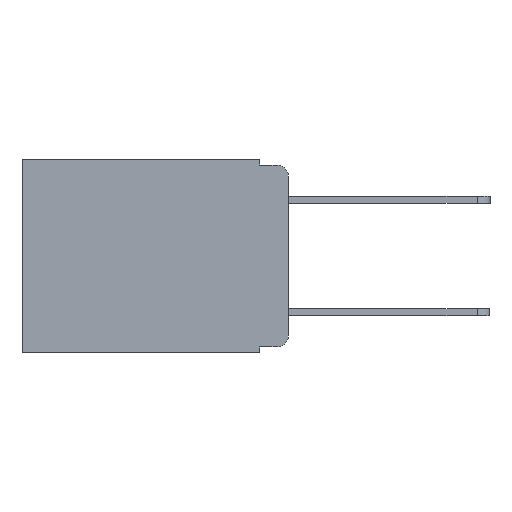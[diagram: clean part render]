
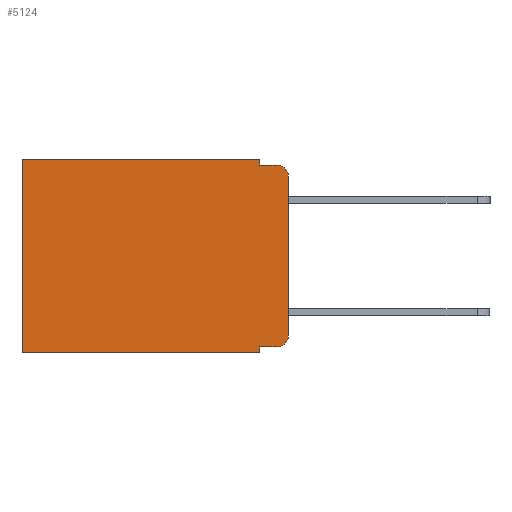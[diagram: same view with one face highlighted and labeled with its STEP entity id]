
A CAD part, left-side view. The second image highlights one B-rep face of the part: STEP entity #5124.
In plain terms, the highlighted planar face has unit normal (-1, 0, 0).
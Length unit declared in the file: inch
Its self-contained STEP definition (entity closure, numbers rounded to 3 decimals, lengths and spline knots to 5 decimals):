
#70 = LINE ( 'NONE', #1626, #19078 ) ;
#464 = ORIENTED_EDGE ( 'NONE', *, *, #7212, .F. ) ;
#590 = CARTESIAN_POINT ( 'NONE',  ( 0.298, 0., 0. ) ) ;
#934 = VERTEX_POINT ( 'NONE', #15939 ) ;
#961 = CIRCLE ( 'NONE', #19125, 0.02 ) ;
#998 = VECTOR ( 'NONE', #14916, 39.37008 ) ;
#1626 = CARTESIAN_POINT ( 'NONE',  ( 0.298, 0.051, -0.01 ) ) ;
#1987 = ORIENTED_EDGE ( 'NONE', *, *, #23330, .T. ) ;
#2326 = VECTOR ( 'NONE', #5516, 39.37008 ) ;
#2401 = CARTESIAN_POINT ( 'NONE',  ( 0.298, 0.02, -0.01 ) ) ;
#2480 = CARTESIAN_POINT ( 'NONE',  ( 0.298, 0.051, -0.343 ) ) ;
#2609 = ORIENTED_EDGE ( 'NONE', *, *, #18792, .T. ) ;
#2703 = EDGE_CURVE ( 'NONE', #2738, #21969, #961, .T. ) ;
#2738 = VERTEX_POINT ( 'NONE', #14246 ) ;
#2859 = CIRCLE ( 'NONE', #20068, 0.02 ) ;
#3215 = ORIENTED_EDGE ( 'NONE', *, *, #3689, .F. ) ;
#3340 = VECTOR ( 'NONE', #21827, 39.37008 ) ;
#3397 = EDGE_CURVE ( 'NONE', #18143, #21969, #20705, .T. ) ;
#3503 = VECTOR ( 'NONE', #4278, 39.37008 ) ;
#3689 = EDGE_CURVE ( 'NONE', #23523, #934, #20412, .T. ) ;
#3880 = ORIENTED_EDGE ( 'NONE', *, *, #3397, .F. ) ;
#3925 = DIRECTION ( 'NONE',  ( 1., 0., 0. ) ) ;
#4140 = ORIENTED_EDGE ( 'NONE', *, *, #2703, .T. ) ;
#4278 = DIRECTION ( 'NONE',  ( 0., 0., -1. ) ) ;
#4550 = LINE ( 'NONE', #5565, #3340 ) ;
#5124 = ADVANCED_FACE ( 'NONE', ( #10447 ), #13289, .F. ) ;
#5516 = DIRECTION ( 'NONE',  ( 0., -1., 0. ) ) ;
#5565 = CARTESIAN_POINT ( 'NONE',  ( 0.298, 0., 0. ) ) ;
#5632 = VECTOR ( 'NONE', #14801, 39.37008 ) ;
#6038 = LINE ( 'NONE', #9409, #998 ) ;
#7212 = EDGE_CURVE ( 'NONE', #16788, #8589, #8350, .T. ) ;
#7279 = LINE ( 'NONE', #18158, #2326 ) ;
#7299 = CARTESIAN_POINT ( 'NONE',  ( 0.298, 0., -0.343 ) ) ;
#8350 = LINE ( 'NONE', #20517, #3503 ) ;
#8589 = VERTEX_POINT ( 'NONE', #16200 ) ;
#8881 = VERTEX_POINT ( 'NONE', #2401 ) ;
#8990 = DIRECTION ( 'NONE',  ( 0., -1., 0. ) ) ;
#9409 = CARTESIAN_POINT ( 'NONE',  ( 0.298, 0.051, 0. ) ) ;
#9480 = ORIENTED_EDGE ( 'NONE', *, *, #17414, .T. ) ;
#9644 = CARTESIAN_POINT ( 'NONE',  ( 0.298, 0., -0.03 ) ) ;
#9775 = DIRECTION ( 'NONE',  ( -1., 0., 0. ) ) ;
#10447 = FACE_OUTER_BOUND ( 'NONE', #13478, .T. ) ;
#10485 = VECTOR ( 'NONE', #17546, 39.37008 ) ;
#10700 = VERTEX_POINT ( 'NONE', #22334 ) ;
#10759 = VECTOR ( 'NONE', #18144, 39.37008 ) ;
#11469 = ORIENTED_EDGE ( 'NONE', *, *, #22650, .T. ) ;
#12740 = CARTESIAN_POINT ( 'NONE',  ( 0.298, 0.051, 0. ) ) ;
#12962 = CARTESIAN_POINT ( 'NONE',  ( 0.298, 0.473, 0. ) ) ;
#13289 = PLANE ( 'NONE',  #20168 ) ;
#13478 = EDGE_LOOP ( 'NONE', ( #3880, #2609, #21661, #464, #11469, #1987, #3215, #20037, #9480, #4140 ) ) ;
#13732 = EDGE_CURVE ( 'NONE', #8589, #8881, #70, .T. ) ;
#13921 = CARTESIAN_POINT ( 'NONE',  ( 0.298, 0., -0.313 ) ) ;
#14246 = CARTESIAN_POINT ( 'NONE',  ( 0.298, 0.02, -0.333 ) ) ;
#14333 = CARTESIAN_POINT ( 'NONE',  ( 0.298, 0., 0. ) ) ;
#14801 = DIRECTION ( 'NONE',  ( 0., 0., -1. ) ) ;
#14916 = DIRECTION ( 'NONE',  ( 0., 0., -1. ) ) ;
#15594 = CARTESIAN_POINT ( 'NONE',  ( 0.298, 0.02, -0.313 ) ) ;
#15939 = CARTESIAN_POINT ( 'NONE',  ( 0.298, 0.473, -0.343 ) ) ;
#16200 = CARTESIAN_POINT ( 'NONE',  ( 0.298, 0.051, -0.01 ) ) ;
#16630 = VERTEX_POINT ( 'NONE', #23133 ) ;
#16788 = VERTEX_POINT ( 'NONE', #12740 ) ;
#17414 = EDGE_CURVE ( 'NONE', #16630, #2738, #7279, .T. ) ;
#17546 = DIRECTION ( 'NONE',  ( 0., 0., -1. ) ) ;
#18143 = VERTEX_POINT ( 'NONE', #9644 ) ;
#18144 = DIRECTION ( 'NONE',  ( 0., 1., 0. ) ) ;
#18158 = CARTESIAN_POINT ( 'NONE',  ( 0.298, 0.051, -0.333 ) ) ;
#18792 = EDGE_CURVE ( 'NONE', #18143, #8881, #2859, .T. ) ;
#18902 = DIRECTION ( 'NONE',  ( -1., 0., 0. ) ) ;
#19038 = DIRECTION ( 'NONE',  ( 0., 0., -1. ) ) ;
#19078 = VECTOR ( 'NONE', #8990, 39.37008 ) ;
#19125 = AXIS2_PLACEMENT_3D ( 'NONE', #15594, #18902, #19038 ) ;
#20037 = ORIENTED_EDGE ( 'NONE', *, *, #20994, .F. ) ;
#20068 = AXIS2_PLACEMENT_3D ( 'NONE', #20657, #9775, #22406 ) ;
#20086 = LINE ( 'NONE', #12962, #5632 ) ;
#20168 = AXIS2_PLACEMENT_3D ( 'NONE', #590, #3925, #21835 ) ;
#20412 = LINE ( 'NONE', #7299, #10759 ) ;
#20517 = CARTESIAN_POINT ( 'NONE',  ( 0.298, 0.051, 0. ) ) ;
#20657 = CARTESIAN_POINT ( 'NONE',  ( 0.298, 0.02, -0.03 ) ) ;
#20705 = LINE ( 'NONE', #14333, #10485 ) ;
#20994 = EDGE_CURVE ( 'NONE', #16630, #23523, #6038, .T. ) ;
#21661 = ORIENTED_EDGE ( 'NONE', *, *, #13732, .F. ) ;
#21827 = DIRECTION ( 'NONE',  ( 0., 1., 0. ) ) ;
#21835 = DIRECTION ( 'NONE',  ( 0., 0., -1. ) ) ;
#21969 = VERTEX_POINT ( 'NONE', #13921 ) ;
#22334 = CARTESIAN_POINT ( 'NONE',  ( 0.298, 0.473, 0. ) ) ;
#22406 = DIRECTION ( 'NONE',  ( 0., 0., -1. ) ) ;
#22650 = EDGE_CURVE ( 'NONE', #16788, #10700, #4550, .T. ) ;
#23133 = CARTESIAN_POINT ( 'NONE',  ( 0.298, 0.051, -0.333 ) ) ;
#23330 = EDGE_CURVE ( 'NONE', #10700, #934, #20086, .T. ) ;
#23523 = VERTEX_POINT ( 'NONE', #2480 ) ;
